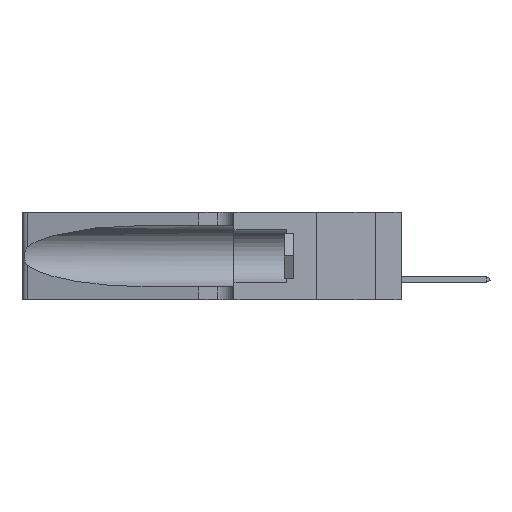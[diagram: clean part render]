
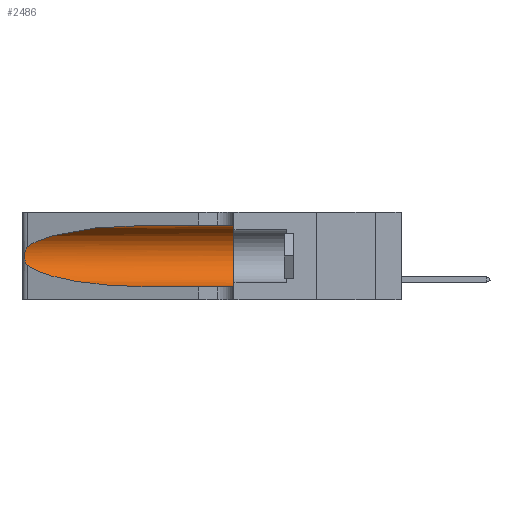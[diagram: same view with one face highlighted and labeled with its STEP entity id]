
A CAD part, left-side view. The second image highlights one B-rep face of the part: STEP entity #2486.
In plain terms, the highlighted cylindrical face has radius 3.308 mm (diameter 6.617 mm), a partial arc.
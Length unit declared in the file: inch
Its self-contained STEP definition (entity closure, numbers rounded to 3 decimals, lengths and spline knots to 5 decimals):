
#1679 = ORIENTED_EDGE ( 'NONE', *, *, #42027, .F. ) ;
#1739 = CARTESIAN_POINT ( 'NONE',  ( 0.1305, 1.61858, 0.05475 ) ) ;
#1850 = FACE_OUTER_BOUND ( 'NONE', #34603, .T. ) ;
#2486 = ADVANCED_FACE ( 'NONE', ( #1850 ), #27712, .F. ) ;
#2732 = CARTESIAN_POINT ( 'NONE',  ( 0.18966, 0.96281, 0.31525 ) ) ;
#2894 = CARTESIAN_POINT ( 'NONE',  ( 0.1305, 0.72297, 0.31525 ) ) ;
#3592 = VERTEX_POINT ( 'NONE', #38282 ) ;
#4526 = LINE ( 'NONE', #27041, #23629 ) ;
#4850 = CARTESIAN_POINT ( 'NONE',  ( 0.1305, 0.35, 0.05475 ) ) ;
#5364 = ORIENTED_EDGE ( 'NONE', *, *, #24038, .T. ) ;
#5583 = CARTESIAN_POINT ( 'NONE',  ( 0.25854, 1.2359, 0.20912 ) ) ;
#5668 = VERTEX_POINT ( 'NONE', #37045 ) ;
#5731 = CARTESIAN_POINT ( 'NONE',  ( 0.25856, 1.23593, 0.16098 ) ) ;
#6010 = VERTEX_POINT ( 'NONE', #43706 ) ;
#6817 = CARTESIAN_POINT ( 'NONE',  ( 0.1305, 0.35, 0.185 ) ) ;
#7809 = CARTESIAN_POINT ( 'NONE',  ( 0.18966, 0.96281, 0.05475 ) ) ;
#8111 = CARTESIAN_POINT ( 'NONE',  ( 0.1305, 0.72297, 0.05475 ) ) ;
#8976 = CARTESIAN_POINT ( 'NONE',  ( 0.26017, 1.23833, 0.17102 ) ) ;
#10271 = AXIS2_PLACEMENT_3D ( 'NONE', #6817, #17060, #40679 ) ;
#10346 = VERTEX_POINT ( 'NONE', #21997 ) ;
#10483 = EDGE_CURVE ( 'NONE', #5668, #6010, #24261, .T. ) ;
#11438 = EDGE_CURVE ( 'NONE', #5668, #22425, #4526, .T. ) ;
#11945 = CARTESIAN_POINT ( 'NONE',  ( 0.26018, 1.23835, 0.19895 ) ) ;
#13549 = DIRECTION ( 'NONE',  ( 0., -1., 0. ) ) ;
#14331 = CARTESIAN_POINT ( 'NONE',  ( 0.2373, 1.15595, 0.08982 ) ) ;
#14751 = DIRECTION ( 'NONE',  ( 0., -1., 0. ) ) ;
#15604 = CARTESIAN_POINT ( 'NONE',  ( 0.1305, 1.61858, 0.185 ) ) ;
#15811 = CARTESIAN_POINT ( 'NONE',  ( 0.25639, 1.23184, 0.21858 ) ) ;
#16482 = DIRECTION ( 'NONE',  ( 0., 0., -1. ) ) ;
#16627 = VECTOR ( 'NONE', #14751, 39.37008 ) ;
#17060 = DIRECTION ( 'NONE',  ( 0., 1., 0. ) ) ;
#18322 =( BOUNDED_CURVE ( )  B_SPLINE_CURVE ( 3, ( #29940, #14331, #7809, #8111 ),
 .UNSPECIFIED., .F., .T. ) 
 B_SPLINE_CURVE_WITH_KNOTS ( ( 4, 4 ),
 ( 3.44316, 4.71239 ),
 .UNSPECIFIED. ) 
 CURVE ( )  GEOMETRIC_REPRESENTATION_ITEM ( )  RATIONAL_B_SPLINE_CURVE ( ( 1., 0.87, 0.87, 1. ) ) 
 REPRESENTATION_ITEM ( '' )  );
#20742 = ORIENTED_EDGE ( 'NONE', *, *, #28360, .T. ) ;
#21997 = CARTESIAN_POINT ( 'NONE',  ( 0.25487, 1.22718, 0.14631 ) ) ;
#22036 = CARTESIAN_POINT ( 'NONE',  ( 0.26075, 1.23896, 0.19203 ) ) ;
#22409 = B_SPLINE_CURVE_WITH_KNOTS ( 'NONE', 3,
 ( #42581, #35768, #15811, #39294, #5583, #11945, #22036, #29103, #8976, #5731, #32662, #39438, #22645, #42878 ),
 .UNSPECIFIED., .F., .F.,
 ( 4, 2, 2, 2, 2, 2, 4 ),
 ( 0., 0.00027, 0.00053, 0.00107, 0.0016, 0.00187, 0.00214 ),
 .UNSPECIFIED. ) ;
#22425 = VERTEX_POINT ( 'NONE', #39640 ) ;
#22645 = CARTESIAN_POINT ( 'NONE',  ( 0.25555, 1.22993, 0.14849 ) ) ;
#23629 = VECTOR ( 'NONE', #13549, 39.37008 ) ;
#24038 = EDGE_CURVE ( 'NONE', #6010, #10346, #22409, .T. ) ;
#24261 =( BOUNDED_CURVE ( )  B_SPLINE_CURVE ( 3, ( #2894, #2732, #30079, #36900 ),
 .UNSPECIFIED., .F., .T. ) 
 B_SPLINE_CURVE_WITH_KNOTS ( ( 4, 4 ),
 ( 1.5708, 2.84003 ),
 .UNSPECIFIED. ) 
 CURVE ( )  GEOMETRIC_REPRESENTATION_ITEM ( )  RATIONAL_B_SPLINE_CURVE ( ( 1., 0.87, 0.87, 1. ) ) 
 REPRESENTATION_ITEM ( '' )  );
#25638 = LINE ( 'NONE', #1739, #16627 ) ;
#26725 = ORIENTED_EDGE ( 'NONE', *, *, #11438, .F. ) ;
#27041 = CARTESIAN_POINT ( 'NONE',  ( 0.1305, 1.61858, 0.31525 ) ) ;
#27712 = CYLINDRICAL_SURFACE ( 'NONE', #36940, 0.13025 ) ;
#28124 = CIRCLE ( 'NONE', #10271, 0.13025 ) ;
#28360 = EDGE_CURVE ( 'NONE', #10346, #3592, #18322, .T. ) ;
#28573 = DIRECTION ( 'NONE',  ( 0., -1., 0. ) ) ;
#29103 = CARTESIAN_POINT ( 'NONE',  ( 0.26075, 1.23896, 0.178 ) ) ;
#29940 = CARTESIAN_POINT ( 'NONE',  ( 0.25487, 1.22718, 0.14631 ) ) ;
#30079 = CARTESIAN_POINT ( 'NONE',  ( 0.2373, 1.15595, 0.28018 ) ) ;
#31236 = ORIENTED_EDGE ( 'NONE', *, *, #10483, .T. ) ;
#32459 = VERTEX_POINT ( 'NONE', #4850 ) ;
#32518 = EDGE_CURVE ( 'NONE', #3592, #32459, #25638, .T. ) ;
#32662 = CARTESIAN_POINT ( 'NONE',  ( 0.25789, 1.23486, 0.15765 ) ) ;
#34603 = EDGE_LOOP ( 'NONE', ( #31236, #5364, #20742, #38437, #1679, #26725 ) ) ;
#35768 = CARTESIAN_POINT ( 'NONE',  ( 0.25555, 1.22994, 0.2215 ) ) ;
#36900 = CARTESIAN_POINT ( 'NONE',  ( 0.25487, 1.22718, 0.22369 ) ) ;
#36940 = AXIS2_PLACEMENT_3D ( 'NONE', #15604, #28573, #16482 ) ;
#37045 = CARTESIAN_POINT ( 'NONE',  ( 0.1305, 0.72297, 0.31525 ) ) ;
#38282 = CARTESIAN_POINT ( 'NONE',  ( 0.1305, 0.72297, 0.05475 ) ) ;
#38437 = ORIENTED_EDGE ( 'NONE', *, *, #32518, .T. ) ;
#39294 = CARTESIAN_POINT ( 'NONE',  ( 0.25787, 1.23484, 0.2124 ) ) ;
#39438 = CARTESIAN_POINT ( 'NONE',  ( 0.25639, 1.23186, 0.15144 ) ) ;
#39640 = CARTESIAN_POINT ( 'NONE',  ( 0.1305, 0.35, 0.31525 ) ) ;
#40679 = DIRECTION ( 'NONE',  ( 0., 0., 1. ) ) ;
#42027 = EDGE_CURVE ( 'NONE', #22425, #32459, #28124, .T. ) ;
#42581 = CARTESIAN_POINT ( 'NONE',  ( 0.25487, 1.22718, 0.22369 ) ) ;
#42878 = CARTESIAN_POINT ( 'NONE',  ( 0.25487, 1.22718, 0.14631 ) ) ;
#43706 = CARTESIAN_POINT ( 'NONE',  ( 0.25487, 1.22718, 0.22369 ) ) ;
